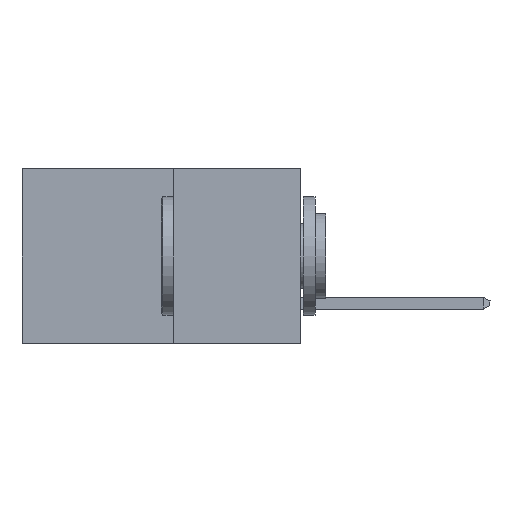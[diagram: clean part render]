
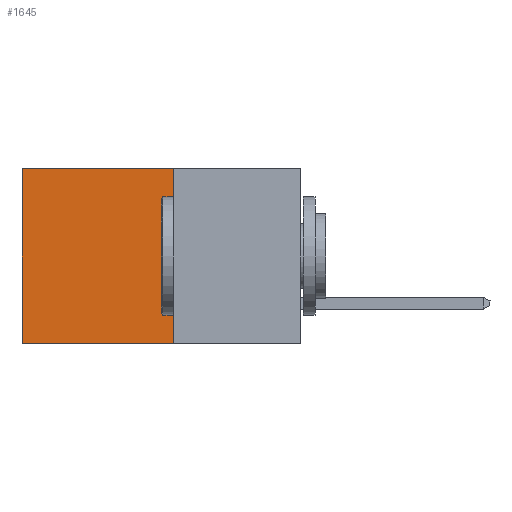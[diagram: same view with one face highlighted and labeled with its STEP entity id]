
A CAD part, left-side view. The second image highlights one B-rep face of the part: STEP entity #1645.
In plain terms, the highlighted planar face has unit normal (-1, 0, 0).
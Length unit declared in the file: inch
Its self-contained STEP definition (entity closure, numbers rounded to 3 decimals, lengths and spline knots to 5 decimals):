
#616 = EDGE_CURVE ( 'NONE', #6689, #12955, #17595, .T. ) ;
#1442 = CARTESIAN_POINT ( 'NONE',  ( 0.277, 0.27, -0.37 ) ) ;
#1645 = ADVANCED_FACE ( 'NONE', ( #18785 ), #1928, .F. ) ;
#1879 = DIRECTION ( 'NONE',  ( 1., 0., 0. ) ) ;
#1928 = PLANE ( 'NONE',  #17489 ) ;
#3111 = VECTOR ( 'NONE', #9769, 39.37008 ) ;
#3324 = EDGE_CURVE ( 'NONE', #7302, #6689, #20229, .T. ) ;
#3669 = CARTESIAN_POINT ( 'NONE',  ( 0.277, 0.27, -0.37 ) ) ;
#3828 = CARTESIAN_POINT ( 'NONE',  ( 0.277, 0.27, 0. ) ) ;
#4006 = CARTESIAN_POINT ( 'NONE',  ( 0.277, 0.27, -0.37 ) ) ;
#5269 = VERTEX_POINT ( 'NONE', #1442 ) ;
#6689 = VERTEX_POINT ( 'NONE', #12762 ) ;
#7302 = VERTEX_POINT ( 'NONE', #3828 ) ;
#8145 = CARTESIAN_POINT ( 'NONE',  ( 0.277, 0.27, -0.37 ) ) ;
#8649 = EDGE_CURVE ( 'NONE', #5269, #12955, #13591, .T. ) ;
#9769 = DIRECTION ( 'NONE',  ( 0., 0., -1. ) ) ;
#10227 = EDGE_CURVE ( 'NONE', #7302, #5269, #20313, .T. ) ;
#11517 = DIRECTION ( 'NONE',  ( 0., 1., 0. ) ) ;
#12762 = CARTESIAN_POINT ( 'NONE',  ( 0.277, 0.59, 0. ) ) ;
#12955 = VERTEX_POINT ( 'NONE', #17008 ) ;
#13305 = VECTOR ( 'NONE', #17495, 39.37008 ) ;
#13591 = LINE ( 'NONE', #4006, #17363 ) ;
#13944 = ORIENTED_EDGE ( 'NONE', *, *, #10227, .F. ) ;
#14669 = DIRECTION ( 'NONE',  ( 0., 0., -1. ) ) ;
#14965 = VECTOR ( 'NONE', #11517, 39.37008 ) ;
#15384 = DIRECTION ( 'NONE',  ( 0., 1., 0. ) ) ;
#15926 = ORIENTED_EDGE ( 'NONE', *, *, #616, .T. ) ;
#16695 = EDGE_LOOP ( 'NONE', ( #15926, #20494, #13944, #17255 ) ) ;
#16844 = CARTESIAN_POINT ( 'NONE',  ( 0.277, 0.59, -0.37 ) ) ;
#17008 = CARTESIAN_POINT ( 'NONE',  ( 0.277, 0.59, -0.37 ) ) ;
#17255 = ORIENTED_EDGE ( 'NONE', *, *, #3324, .T. ) ;
#17363 = VECTOR ( 'NONE', #15384, 39.37008 ) ;
#17369 = CARTESIAN_POINT ( 'NONE',  ( 0.277, 0.27, 0. ) ) ;
#17489 = AXIS2_PLACEMENT_3D ( 'NONE', #3669, #1879, #14669 ) ;
#17495 = DIRECTION ( 'NONE',  ( 0., 0., -1. ) ) ;
#17595 = LINE ( 'NONE', #16844, #13305 ) ;
#18785 = FACE_OUTER_BOUND ( 'NONE', #16695, .T. ) ;
#20229 = LINE ( 'NONE', #17369, #14965 ) ;
#20313 = LINE ( 'NONE', #8145, #3111 ) ;
#20494 = ORIENTED_EDGE ( 'NONE', *, *, #8649, .F. ) ;
